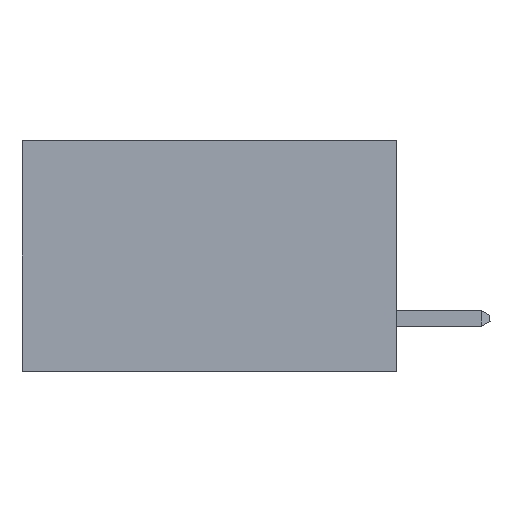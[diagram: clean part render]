
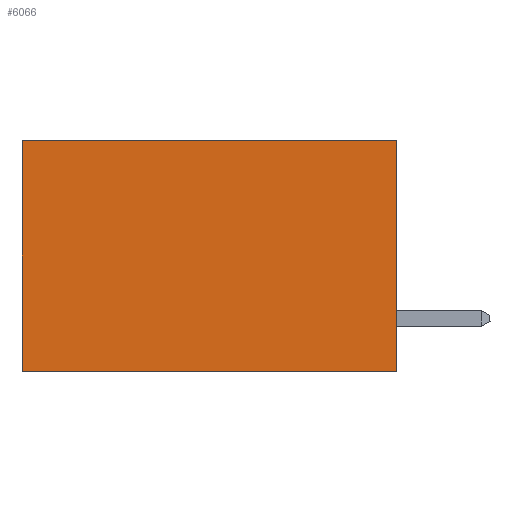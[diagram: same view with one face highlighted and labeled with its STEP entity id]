
A CAD part, left-side view. The second image highlights one B-rep face of the part: STEP entity #6066.
In plain terms, the highlighted planar face has unit normal (-1, 0, 0).
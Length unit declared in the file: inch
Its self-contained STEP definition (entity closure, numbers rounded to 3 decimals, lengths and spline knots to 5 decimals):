
#170 = DIRECTION ( 'NONE',  ( 0., 1., 0. ) ) ;
#951 = LINE ( 'NONE', #17662, #14862 ) ;
#1899 = EDGE_CURVE ( 'NONE', #22742, #8562, #5098, .T. ) ;
#2178 = CARTESIAN_POINT ( 'NONE',  ( 0.298, 0.6, -0.37 ) ) ;
#2639 = EDGE_CURVE ( 'NONE', #12324, #20152, #13048, .T. ) ;
#2921 = FACE_OUTER_BOUND ( 'NONE', #11193, .T. ) ;
#2991 = VECTOR ( 'NONE', #3328, 39.37008 ) ;
#3328 = DIRECTION ( 'NONE',  ( 0., 1., 0. ) ) ;
#5098 = LINE ( 'NONE', #8311, #14589 ) ;
#5206 = ORIENTED_EDGE ( 'NONE', *, *, #1899, .F. ) ;
#5358 = ORIENTED_EDGE ( 'NONE', *, *, #10599, .F. ) ;
#6066 = ADVANCED_FACE ( 'NONE', ( #2921 ), #9921, .F. ) ;
#7014 = CARTESIAN_POINT ( 'NONE',  ( 0.298, 0., 0. ) ) ;
#7675 = CARTESIAN_POINT ( 'NONE',  ( 0.298, 0., 0. ) ) ;
#8089 = ORIENTED_EDGE ( 'NONE', *, *, #2639, .T. ) ;
#8311 = CARTESIAN_POINT ( 'NONE',  ( 0.298, 0., -0.37 ) ) ;
#8562 = VERTEX_POINT ( 'NONE', #2178 ) ;
#8645 = EDGE_CURVE ( 'NONE', #20152, #8562, #17857, .T. ) ;
#9918 = CARTESIAN_POINT ( 'NONE',  ( 0.298, 0., -0.37 ) ) ;
#9921 = PLANE ( 'NONE',  #22384 ) ;
#10599 = EDGE_CURVE ( 'NONE', #12324, #22742, #951, .T. ) ;
#11193 = EDGE_LOOP ( 'NONE', ( #13289, #5206, #5358, #8089 ) ) ;
#12324 = VERTEX_POINT ( 'NONE', #7675 ) ;
#12919 = CARTESIAN_POINT ( 'NONE',  ( 0.298, 0., 0. ) ) ;
#13048 = LINE ( 'NONE', #12919, #2991 ) ;
#13289 = ORIENTED_EDGE ( 'NONE', *, *, #8645, .T. ) ;
#14589 = VECTOR ( 'NONE', #170, 39.37008 ) ;
#14862 = VECTOR ( 'NONE', #19488, 39.37008 ) ;
#15657 = DIRECTION ( 'NONE',  ( 0., 0., -1. ) ) ;
#16664 = DIRECTION ( 'NONE',  ( 0., 0., -1. ) ) ;
#17266 = VECTOR ( 'NONE', #15657, 39.37008 ) ;
#17662 = CARTESIAN_POINT ( 'NONE',  ( 0.298, 0., 0. ) ) ;
#17857 = LINE ( 'NONE', #19370, #17266 ) ;
#18478 = CARTESIAN_POINT ( 'NONE',  ( 0.298, 0.6, 0. ) ) ;
#19370 = CARTESIAN_POINT ( 'NONE',  ( 0.298, 0.6, 0. ) ) ;
#19483 = DIRECTION ( 'NONE',  ( 1., 0., 0. ) ) ;
#19488 = DIRECTION ( 'NONE',  ( 0., 0., -1. ) ) ;
#20152 = VERTEX_POINT ( 'NONE', #18478 ) ;
#22384 = AXIS2_PLACEMENT_3D ( 'NONE', #7014, #19483, #16664 ) ;
#22742 = VERTEX_POINT ( 'NONE', #9918 ) ;
